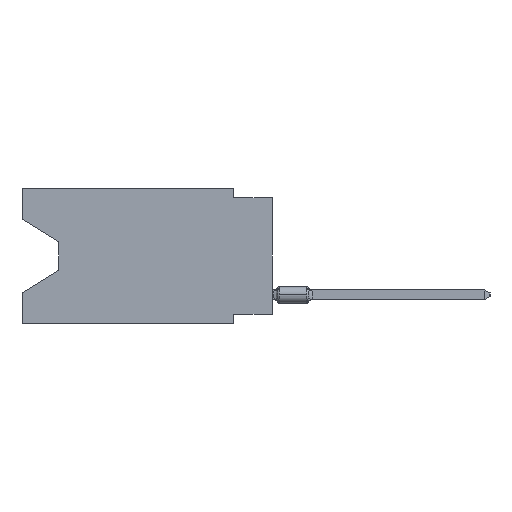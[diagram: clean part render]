
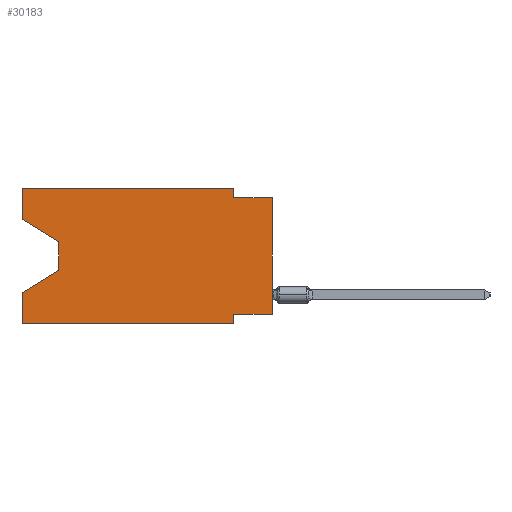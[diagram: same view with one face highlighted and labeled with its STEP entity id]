
A CAD part, left-side view. The second image highlights one B-rep face of the part: STEP entity #30183.
In plain terms, the highlighted planar face has unit normal (-1, 0, 0).
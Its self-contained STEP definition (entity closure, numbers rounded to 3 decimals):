
#121 = ORIENTED_EDGE ( 'NONE', *, *, #9178, .T. ) ;
#212 = CARTESIAN_POINT ( 'NONE',  ( 0., 2.54, -0.635 ) ) ;
#487 = VECTOR ( 'NONE', #1768, 1000. ) ;
#1319 = VERTEX_POINT ( 'NONE', #18028 ) ;
#1391 = EDGE_CURVE ( 'NONE', #19333, #22795, #4551, .T. ) ;
#1635 = ORIENTED_EDGE ( 'NONE', *, *, #20105, .T. ) ;
#1768 = DIRECTION ( 'NONE',  ( 0., 0., 1. ) ) ;
#2386 = CARTESIAN_POINT ( 'NONE',  ( 0., 13.97, -3.505 ) ) ;
#2491 = VECTOR ( 'NONE', #26226, 1000. ) ;
#3188 = CARTESIAN_POINT ( 'NONE',  ( 0., 16.383, -2.038 ) ) ;
#3934 = VECTOR ( 'NONE', #43361, 1000. ) ;
#4093 = CARTESIAN_POINT ( 'NONE',  ( 0., 16.383, 0. ) ) ;
#4551 = LINE ( 'NONE', #11534, #2491 ) ;
#4944 = VERTEX_POINT ( 'NONE', #42354 ) ;
#5040 = ORIENTED_EDGE ( 'NONE', *, *, #1391, .T. ) ;
#5863 = ORIENTED_EDGE ( 'NONE', *, *, #26073, .F. ) ;
#6531 = FACE_OUTER_BOUND ( 'NONE', #45576, .T. ) ;
#7701 = LINE ( 'NONE', #26698, #31813 ) ;
#8720 = VERTEX_POINT ( 'NONE', #42578 ) ;
#9178 = EDGE_CURVE ( 'NONE', #22795, #4944, #16539, .T. ) ;
#9340 = LINE ( 'NONE', #35071, #47296 ) ;
#9568 = DIRECTION ( 'NONE',  ( 0., 0.855, -0.519 ) ) ;
#10084 = VECTOR ( 'NONE', #43525, 1000. ) ;
#11534 = CARTESIAN_POINT ( 'NONE',  ( 0., 13.97, -3.505 ) ) ;
#12395 = VECTOR ( 'NONE', #20478, 1000. ) ;
#12696 = DIRECTION ( 'NONE',  ( 0., 0., 1. ) ) ;
#12862 = VECTOR ( 'NONE', #38830, 1000. ) ;
#13506 = LINE ( 'NONE', #27982, #487 ) ;
#13991 = CARTESIAN_POINT ( 'NONE',  ( 0., 16.383, 0. ) ) ;
#14226 = CARTESIAN_POINT ( 'NONE',  ( 0., 0., -8.255 ) ) ;
#15561 = EDGE_CURVE ( 'NONE', #42506, #8720, #24160, .T. ) ;
#16539 = LINE ( 'NONE', #20641, #40423 ) ;
#16607 = EDGE_CURVE ( 'NONE', #1319, #42154, #38535, .T. ) ;
#17395 = LINE ( 'NONE', #32089, #12862 ) ;
#17609 = PLANE ( 'NONE',  #36820 ) ;
#17652 = DIRECTION ( 'NONE',  ( 0., -1., 0. ) ) ;
#18008 = EDGE_CURVE ( 'NONE', #27042, #31663, #27482, .T. ) ;
#18028 = CARTESIAN_POINT ( 'NONE',  ( 0., 16.383, -8.89 ) ) ;
#18116 = EDGE_CURVE ( 'NONE', #1319, #4944, #22379, .T. ) ;
#19333 = VERTEX_POINT ( 'NONE', #2386 ) ;
#19770 = VERTEX_POINT ( 'NONE', #33335 ) ;
#20105 = EDGE_CURVE ( 'NONE', #46098, #19333, #17395, .T. ) ;
#20433 = ORIENTED_EDGE ( 'NONE', *, *, #46054, .T. ) ;
#20478 = DIRECTION ( 'NONE',  ( 0., 1., 0. ) ) ;
#20641 = CARTESIAN_POINT ( 'NONE',  ( 0., 13.97, -5.385 ) ) ;
#22379 = LINE ( 'NONE', #4093, #10084 ) ;
#22795 = VERTEX_POINT ( 'NONE', #41927 ) ;
#23094 = LINE ( 'NONE', #27196, #35254 ) ;
#23318 = DIRECTION ( 'NONE',  ( 0., -1., 0. ) ) ;
#24160 = LINE ( 'NONE', #42659, #26078 ) ;
#25055 = DIRECTION ( 'NONE',  ( 0., 0., -1. ) ) ;
#25096 = CARTESIAN_POINT ( 'NONE',  ( 0., 2.54, -8.89 ) ) ;
#25100 = ORIENTED_EDGE ( 'NONE', *, *, #15561, .F. ) ;
#26073 = EDGE_CURVE ( 'NONE', #31663, #42154, #35917, .T. ) ;
#26078 = VECTOR ( 'NONE', #17652, 1000. ) ;
#26148 = VECTOR ( 'NONE', #35397, 1000. ) ;
#26226 = DIRECTION ( 'NONE',  ( 0., 0., -1. ) ) ;
#26698 = CARTESIAN_POINT ( 'NONE',  ( 0., 16.383, 0. ) ) ;
#27042 = VERTEX_POINT ( 'NONE', #14226 ) ;
#27196 = CARTESIAN_POINT ( 'NONE',  ( 0., 2.54, 0. ) ) ;
#27482 = LINE ( 'NONE', #43070, #12395 ) ;
#27982 = CARTESIAN_POINT ( 'NONE',  ( 0., 0., 0. ) ) ;
#28685 = DIRECTION ( 'NONE',  ( 1., 0., 0. ) ) ;
#28711 = CARTESIAN_POINT ( 'NONE',  ( 0., 2.54, 0. ) ) ;
#29700 = CARTESIAN_POINT ( 'NONE',  ( 0., 2.54, -8.255 ) ) ;
#30183 = ADVANCED_FACE ( 'NONE', ( #6531 ), #17609, .F. ) ;
#31663 = VERTEX_POINT ( 'NONE', #29700 ) ;
#31813 = VECTOR ( 'NONE', #23318, 1000. ) ;
#32089 = CARTESIAN_POINT ( 'NONE',  ( 0., 16.383, -2.038 ) ) ;
#33335 = CARTESIAN_POINT ( 'NONE',  ( 0., 16.383, 0. ) ) ;
#33564 = ORIENTED_EDGE ( 'NONE', *, *, #42087, .F. ) ;
#35071 = CARTESIAN_POINT ( 'NONE',  ( 0., 16.383, 0. ) ) ;
#35254 = VECTOR ( 'NONE', #41825, 1000. ) ;
#35261 = ORIENTED_EDGE ( 'NONE', *, *, #35588, .F. ) ;
#35397 = DIRECTION ( 'NONE',  ( 0., -1., 0. ) ) ;
#35588 = EDGE_CURVE ( 'NONE', #46098, #19770, #9340, .T. ) ;
#35917 = LINE ( 'NONE', #25096, #3934 ) ;
#36820 = AXIS2_PLACEMENT_3D ( 'NONE', #13991, #28685, #25055 ) ;
#37269 = CARTESIAN_POINT ( 'NONE',  ( 0., 2.54, -8.89 ) ) ;
#37299 = ORIENTED_EDGE ( 'NONE', *, *, #39095, .F. ) ;
#38535 = LINE ( 'NONE', #38761, #26148 ) ;
#38761 = CARTESIAN_POINT ( 'NONE',  ( 0., 16.383, -8.89 ) ) ;
#38830 = DIRECTION ( 'NONE',  ( 0., -0.855, -0.519 ) ) ;
#39095 = EDGE_CURVE ( 'NONE', #41502, #42506, #23094, .T. ) ;
#40423 = VECTOR ( 'NONE', #9568, 1000. ) ;
#41502 = VERTEX_POINT ( 'NONE', #28711 ) ;
#41825 = DIRECTION ( 'NONE',  ( 0., 0., -1. ) ) ;
#41927 = CARTESIAN_POINT ( 'NONE',  ( 0., 13.97, -5.385 ) ) ;
#42087 = EDGE_CURVE ( 'NONE', #19770, #41502, #7701, .T. ) ;
#42154 = VERTEX_POINT ( 'NONE', #37269 ) ;
#42354 = CARTESIAN_POINT ( 'NONE',  ( 0., 16.383, -6.852 ) ) ;
#42506 = VERTEX_POINT ( 'NONE', #212 ) ;
#42578 = CARTESIAN_POINT ( 'NONE',  ( 0., 0., -0.635 ) ) ;
#42659 = CARTESIAN_POINT ( 'NONE',  ( 0., 0., -0.635 ) ) ;
#43070 = CARTESIAN_POINT ( 'NONE',  ( 0., 0., -8.255 ) ) ;
#43361 = DIRECTION ( 'NONE',  ( 0., 0., -1. ) ) ;
#43525 = DIRECTION ( 'NONE',  ( 0., 0., 1. ) ) ;
#43906 = ORIENTED_EDGE ( 'NONE', *, *, #18116, .F. ) ;
#45413 = ORIENTED_EDGE ( 'NONE', *, *, #18008, .F. ) ;
#45435 = ORIENTED_EDGE ( 'NONE', *, *, #16607, .T. ) ;
#45576 = EDGE_LOOP ( 'NONE', ( #1635, #5040, #121, #43906, #45435, #5863, #45413, #20433, #25100, #37299, #33564, #35261 ) ) ;
#46054 = EDGE_CURVE ( 'NONE', #27042, #8720, #13506, .T. ) ;
#46098 = VERTEX_POINT ( 'NONE', #3188 ) ;
#47296 = VECTOR ( 'NONE', #12696, 1000. ) ;
